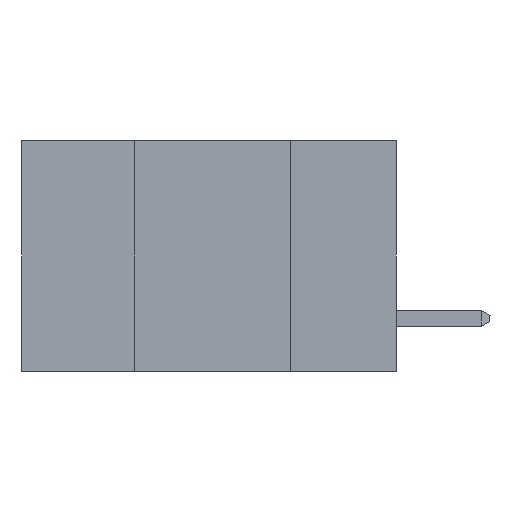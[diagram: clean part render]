
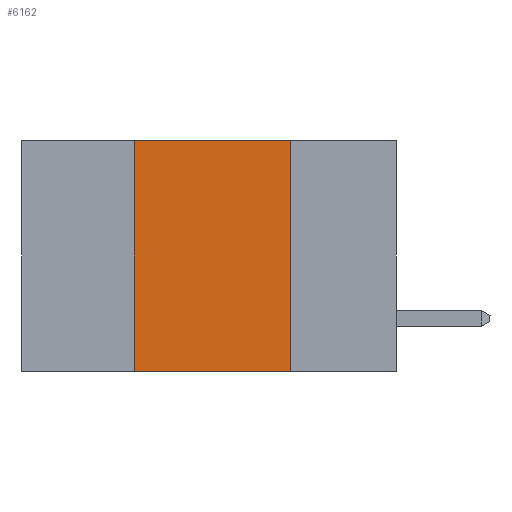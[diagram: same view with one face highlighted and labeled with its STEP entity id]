
A CAD part, left-side view. The second image highlights one B-rep face of the part: STEP entity #6162.
In plain terms, the highlighted planar face has unit normal (-1, 0, 0).
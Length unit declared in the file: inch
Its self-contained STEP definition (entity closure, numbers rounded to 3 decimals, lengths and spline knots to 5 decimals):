
#163 = DIRECTION ( 'NONE',  ( 0., 0., -1. ) ) ;
#758 = LINE ( 'NONE', #13447, #14384 ) ;
#1849 = ORIENTED_EDGE ( 'NONE', *, *, #13164, .F. ) ;
#2640 = CARTESIAN_POINT ( 'NONE',  ( 0., 0.42, -0.37 ) ) ;
#2894 = CARTESIAN_POINT ( 'NONE',  ( 0., 0.42, -0.37 ) ) ;
#2999 = ORIENTED_EDGE ( 'NONE', *, *, #11193, .F. ) ;
#3796 = PLANE ( 'NONE',  #16718 ) ;
#4562 = ORIENTED_EDGE ( 'NONE', *, *, #12556, .F. ) ;
#4741 = LINE ( 'NONE', #21787, #10721 ) ;
#5344 = ORIENTED_EDGE ( 'NONE', *, *, #8462, .T. ) ;
#6162 = ADVANCED_FACE ( 'NONE', ( #13477 ), #3796, .F. ) ;
#6564 = CARTESIAN_POINT ( 'NONE',  ( 0., 0.42, 0. ) ) ;
#7199 = VERTEX_POINT ( 'NONE', #2640 ) ;
#7462 = VECTOR ( 'NONE', #23430, 39.37008 ) ;
#7832 = DIRECTION ( 'NONE',  ( 0., 0., -1. ) ) ;
#7978 = CARTESIAN_POINT ( 'NONE',  ( 0., 0.17, 0. ) ) ;
#8462 = EDGE_CURVE ( 'NONE', #7199, #9960, #4741, .T. ) ;
#9275 = CARTESIAN_POINT ( 'NONE',  ( 0., 0.17, -0.37 ) ) ;
#9856 = VERTEX_POINT ( 'NONE', #6564 ) ;
#9960 = VERTEX_POINT ( 'NONE', #9275 ) ;
#10688 = CARTESIAN_POINT ( 'NONE',  ( 0., 0.6, 0. ) ) ;
#10721 = VECTOR ( 'NONE', #14417, 39.37008 ) ;
#11193 = EDGE_CURVE ( 'NONE', #19508, #9960, #758, .T. ) ;
#11395 = DIRECTION ( 'NONE',  ( 1., 0., 0. ) ) ;
#12556 = EDGE_CURVE ( 'NONE', #7199, #9856, #21557, .T. ) ;
#12570 = LINE ( 'NONE', #10688, #17472 ) ;
#13164 = EDGE_CURVE ( 'NONE', #9856, #19508, #12570, .T. ) ;
#13240 = CARTESIAN_POINT ( 'NONE',  ( 0., 0.6, 0. ) ) ;
#13447 = CARTESIAN_POINT ( 'NONE',  ( 0., 0.17, -0.37 ) ) ;
#13477 = FACE_OUTER_BOUND ( 'NONE', #14111, .T. ) ;
#14111 = EDGE_LOOP ( 'NONE', ( #2999, #1849, #4562, #5344 ) ) ;
#14384 = VECTOR ( 'NONE', #7832, 39.37008 ) ;
#14417 = DIRECTION ( 'NONE',  ( 0., -1., 0. ) ) ;
#16718 = AXIS2_PLACEMENT_3D ( 'NONE', #13240, #11395, #163 ) ;
#17472 = VECTOR ( 'NONE', #18302, 39.37008 ) ;
#18302 = DIRECTION ( 'NONE',  ( 0., -1., 0. ) ) ;
#19508 = VERTEX_POINT ( 'NONE', #7978 ) ;
#21557 = LINE ( 'NONE', #2894, #7462 ) ;
#21787 = CARTESIAN_POINT ( 'NONE',  ( 0., 0.6, -0.37 ) ) ;
#23430 = DIRECTION ( 'NONE',  ( 0., 0., 1. ) ) ;
